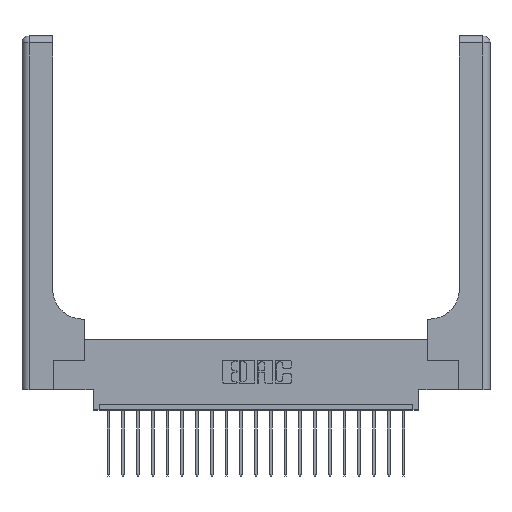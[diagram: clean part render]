
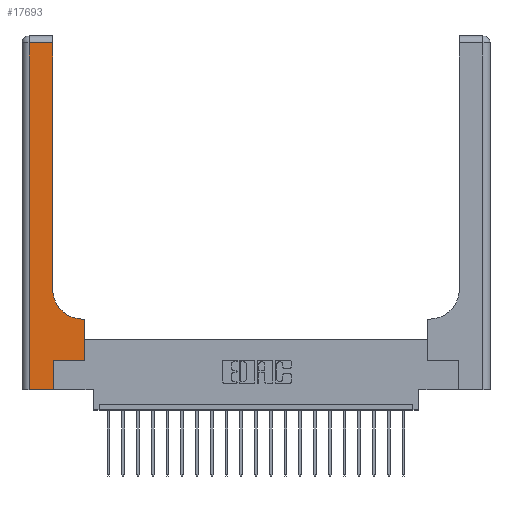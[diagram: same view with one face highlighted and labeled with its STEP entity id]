
A CAD part, top view. The second image highlights one B-rep face of the part: STEP entity #17693.
In plain terms, the highlighted planar face has unit normal (0, 0, 1).
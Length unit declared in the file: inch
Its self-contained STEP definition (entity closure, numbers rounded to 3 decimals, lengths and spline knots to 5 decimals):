
#348 = LINE ( 'NONE', #20724, #20051 ) ;
#441 = DIRECTION ( 'NONE',  ( 0., 1., 0. ) ) ;
#468 = VERTEX_POINT ( 'NONE', #8960 ) ;
#1225 = EDGE_CURVE ( 'NONE', #5969, #6497, #348, .T. ) ;
#1339 = DIRECTION ( 'NONE',  ( -1., 0., 0. ) ) ;
#1668 = FACE_OUTER_BOUND ( 'NONE', #5835, .T. ) ;
#1689 = VECTOR ( 'NONE', #7218, 39.37008 ) ;
#1727 = DIRECTION ( 'NONE',  ( 1., 0., 0. ) ) ;
#1886 = DIRECTION ( 'NONE',  ( -1., 0., 0. ) ) ;
#2067 = EDGE_CURVE ( 'NONE', #9558, #5969, #11071, .T. ) ;
#2359 = ORIENTED_EDGE ( 'NONE', *, *, #2067, .T. ) ;
#2575 = VERTEX_POINT ( 'NONE', #19692 ) ;
#2857 = CARTESIAN_POINT ( 'NONE',  ( 0.06, 0., 0.37 ) ) ;
#3496 = VECTOR ( 'NONE', #1886, 39.37008 ) ;
#3505 = CARTESIAN_POINT ( 'NONE',  ( 0.06, 3., 0.37 ) ) ;
#4174 = VERTEX_POINT ( 'NONE', #2857 ) ;
#4314 = CARTESIAN_POINT ( 'NONE',  ( 0.51, 0.6, 0.37 ) ) ;
#4321 = CARTESIAN_POINT ( 'NONE',  ( 0., 3., 0.37 ) ) ;
#4342 = DIRECTION ( 'NONE',  ( -1., 0., 0. ) ) ;
#4557 = EDGE_CURVE ( 'NONE', #4174, #2575, #8136, .T. ) ;
#4935 = DIRECTION ( 'NONE',  ( 0., 0., -1. ) ) ;
#5297 = DIRECTION ( 'NONE',  ( 0., 1., 0. ) ) ;
#5431 = CARTESIAN_POINT ( 'NONE',  ( 0.528, 0.25, 0.37 ) ) ;
#5473 = ORIENTED_EDGE ( 'NONE', *, *, #20931, .T. ) ;
#5659 = LINE ( 'NONE', #13026, #13868 ) ;
#5835 = EDGE_LOOP ( 'NONE', ( #18123, #17749, #10902, #14447, #5473, #20336, #2359, #15735, #5849 ) ) ;
#5849 = ORIENTED_EDGE ( 'NONE', *, *, #12597, .T. ) ;
#5969 = VERTEX_POINT ( 'NONE', #18499 ) ;
#6374 = LINE ( 'NONE', #3505, #12505 ) ;
#6497 = VERTEX_POINT ( 'NONE', #4314 ) ;
#6983 = DIRECTION ( 'NONE',  ( 1., 0., 0. ) ) ;
#7218 = DIRECTION ( 'NONE',  ( 0., 1., 0. ) ) ;
#7620 = EDGE_CURVE ( 'NONE', #17963, #9558, #5659, .T. ) ;
#8136 = LINE ( 'NONE', #10284, #10970 ) ;
#8363 = VECTOR ( 'NONE', #441, 39.37008 ) ;
#8873 = LINE ( 'NONE', #13262, #3496 ) ;
#8960 = CARTESIAN_POINT ( 'NONE',  ( 0.06, 2.94, 0.37 ) ) ;
#9275 = VECTOR ( 'NONE', #5297, 39.37008 ) ;
#9334 = EDGE_CURVE ( 'NONE', #468, #4174, #6374, .T. ) ;
#9558 = VERTEX_POINT ( 'NONE', #20706 ) ;
#9929 = AXIS2_PLACEMENT_3D ( 'NONE', #14605, #4935, #17804 ) ;
#10284 = CARTESIAN_POINT ( 'NONE',  ( 0., 0., 0.37 ) ) ;
#10305 = DIRECTION ( 'NONE',  ( 0., -1., 0. ) ) ;
#10902 = ORIENTED_EDGE ( 'NONE', *, *, #9334, .T. ) ;
#10970 = VECTOR ( 'NONE', #6983, 39.37008 ) ;
#11071 = LINE ( 'NONE', #5431, #9275 ) ;
#12309 = CARTESIAN_POINT ( 'NONE',  ( 0.26, 2.94, 0.37 ) ) ;
#12505 = VECTOR ( 'NONE', #10305, 39.37008 ) ;
#12527 = CARTESIAN_POINT ( 'NONE',  ( 0.26, 0.85, 0.37 ) ) ;
#12597 = EDGE_CURVE ( 'NONE', #6497, #18357, #13652, .T. ) ;
#12719 = LINE ( 'NONE', #13411, #8363 ) ;
#13026 = CARTESIAN_POINT ( 'NONE',  ( 0.265, 0.25, 0.37 ) ) ;
#13262 = CARTESIAN_POINT ( 'NONE',  ( 0., 2.94, 0.37 ) ) ;
#13411 = CARTESIAN_POINT ( 'NONE',  ( 0.26, 3., 0.37 ) ) ;
#13652 = CIRCLE ( 'NONE', #9929, 0.25 ) ;
#13868 = VECTOR ( 'NONE', #1727, 39.37008 ) ;
#14447 = ORIENTED_EDGE ( 'NONE', *, *, #4557, .T. ) ;
#14605 = CARTESIAN_POINT ( 'NONE',  ( 0.51, 0.85, 0.37 ) ) ;
#14949 = CARTESIAN_POINT ( 'NONE',  ( 0.265, 0.25, 0.37 ) ) ;
#15735 = ORIENTED_EDGE ( 'NONE', *, *, #1225, .T. ) ;
#16024 = DIRECTION ( 'NONE',  ( 0., 0., -1. ) ) ;
#16469 = AXIS2_PLACEMENT_3D ( 'NONE', #4321, #16024, #1339 ) ;
#16727 = EDGE_CURVE ( 'NONE', #21059, #468, #8873, .T. ) ;
#16786 = EDGE_CURVE ( 'NONE', #18357, #21059, #12719, .T. ) ;
#17268 = LINE ( 'NONE', #20307, #1689 ) ;
#17693 = ADVANCED_FACE ( 'NONE', ( #1668 ), #19283, .F. ) ;
#17749 = ORIENTED_EDGE ( 'NONE', *, *, #16727, .T. ) ;
#17804 = DIRECTION ( 'NONE',  ( 1., 0., 0. ) ) ;
#17963 = VERTEX_POINT ( 'NONE', #14949 ) ;
#18123 = ORIENTED_EDGE ( 'NONE', *, *, #16786, .T. ) ;
#18357 = VERTEX_POINT ( 'NONE', #12527 ) ;
#18499 = CARTESIAN_POINT ( 'NONE',  ( 0.528, 0.6, 0.37 ) ) ;
#19283 = PLANE ( 'NONE',  #16469 ) ;
#19692 = CARTESIAN_POINT ( 'NONE',  ( 0.265, 0., 0.37 ) ) ;
#20051 = VECTOR ( 'NONE', #4342, 39.37008 ) ;
#20307 = CARTESIAN_POINT ( 'NONE',  ( 0.265, 0., 0.37 ) ) ;
#20336 = ORIENTED_EDGE ( 'NONE', *, *, #7620, .T. ) ;
#20706 = CARTESIAN_POINT ( 'NONE',  ( 0.528, 0.25, 0.37 ) ) ;
#20724 = CARTESIAN_POINT ( 'NONE',  ( 0.26, 0.6, 0.37 ) ) ;
#20931 = EDGE_CURVE ( 'NONE', #2575, #17963, #17268, .T. ) ;
#21059 = VERTEX_POINT ( 'NONE', #12309 ) ;
